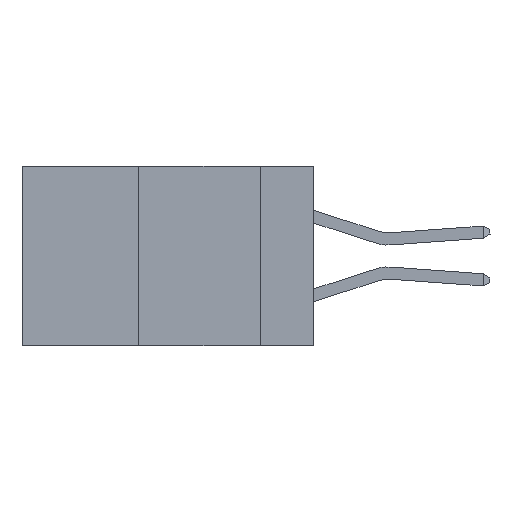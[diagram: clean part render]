
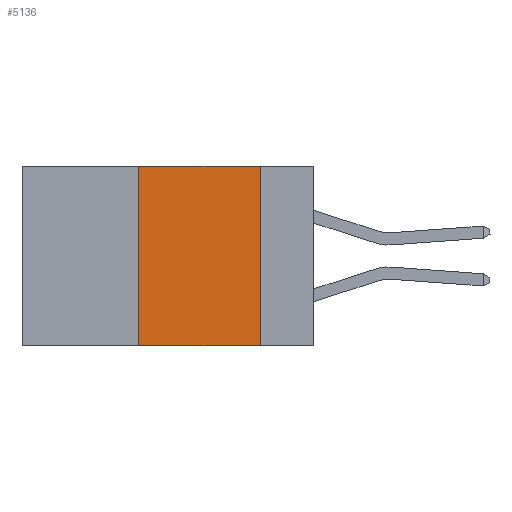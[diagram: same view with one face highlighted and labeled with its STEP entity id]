
A CAD part, left-side view. The second image highlights one B-rep face of the part: STEP entity #5136.
In plain terms, the highlighted planar face has unit normal (-1, 0, 0).
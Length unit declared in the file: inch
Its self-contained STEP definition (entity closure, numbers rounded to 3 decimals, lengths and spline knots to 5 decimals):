
#1392 = FACE_OUTER_BOUND ( 'NONE', #5203, .T. ) ;
#1808 = VECTOR ( 'NONE', #5951, 39.37008 ) ;
#2015 = CARTESIAN_POINT ( 'NONE',  ( 0., 0.36, 0. ) ) ;
#2326 = EDGE_CURVE ( 'NONE', #4226, #9728, #9753, .T. ) ;
#2913 = LINE ( 'NONE', #19272, #1808 ) ;
#4226 = VERTEX_POINT ( 'NONE', #6621 ) ;
#5136 = ADVANCED_FACE ( 'NONE', ( #1392 ), #7954, .F. ) ;
#5201 = DIRECTION ( 'NONE',  ( 0., 0., -1. ) ) ;
#5203 = EDGE_LOOP ( 'NONE', ( #10334, #20547, #15206, #20160 ) ) ;
#5860 = DIRECTION ( 'NONE',  ( 0., -1., 0. ) ) ;
#5951 = DIRECTION ( 'NONE',  ( 0., -1., 0. ) ) ;
#5978 = LINE ( 'NONE', #19098, #11029 ) ;
#6621 = CARTESIAN_POINT ( 'NONE',  ( 0., 0.36, -0.37 ) ) ;
#6766 = DIRECTION ( 'NONE',  ( 0., 0., 1. ) ) ;
#7954 = PLANE ( 'NONE',  #8357 ) ;
#8357 = AXIS2_PLACEMENT_3D ( 'NONE', #14488, #17845, #17964 ) ;
#8436 = VECTOR ( 'NONE', #5201, 39.37008 ) ;
#9728 = VERTEX_POINT ( 'NONE', #2015 ) ;
#9745 = VERTEX_POINT ( 'NONE', #10160 ) ;
#9753 = LINE ( 'NONE', #19463, #14861 ) ;
#10160 = CARTESIAN_POINT ( 'NONE',  ( 0., 0.11, 0. ) ) ;
#10334 = ORIENTED_EDGE ( 'NONE', *, *, #15517, .F. ) ;
#10816 = CARTESIAN_POINT ( 'NONE',  ( 0., 0.11, -0.37 ) ) ;
#11029 = VECTOR ( 'NONE', #5860, 39.37008 ) ;
#12029 = EDGE_CURVE ( 'NONE', #9728, #9745, #5978, .T. ) ;
#12555 = EDGE_CURVE ( 'NONE', #4226, #16120, #2913, .T. ) ;
#14488 = CARTESIAN_POINT ( 'NONE',  ( 0., 0.6, 0. ) ) ;
#14861 = VECTOR ( 'NONE', #6766, 39.37008 ) ;
#15206 = ORIENTED_EDGE ( 'NONE', *, *, #2326, .F. ) ;
#15517 = EDGE_CURVE ( 'NONE', #9745, #16120, #18759, .T. ) ;
#16120 = VERTEX_POINT ( 'NONE', #10816 ) ;
#17128 = CARTESIAN_POINT ( 'NONE',  ( 0., 0.11, 0. ) ) ;
#17845 = DIRECTION ( 'NONE',  ( 1., 0., 0. ) ) ;
#17964 = DIRECTION ( 'NONE',  ( 0., 0., -1. ) ) ;
#18759 = LINE ( 'NONE', #17128, #8436 ) ;
#19098 = CARTESIAN_POINT ( 'NONE',  ( 0., 0.6, 0. ) ) ;
#19272 = CARTESIAN_POINT ( 'NONE',  ( 0., 0.6, -0.37 ) ) ;
#19463 = CARTESIAN_POINT ( 'NONE',  ( 0., 0.36, 0. ) ) ;
#20160 = ORIENTED_EDGE ( 'NONE', *, *, #12555, .T. ) ;
#20547 = ORIENTED_EDGE ( 'NONE', *, *, #12029, .F. ) ;
